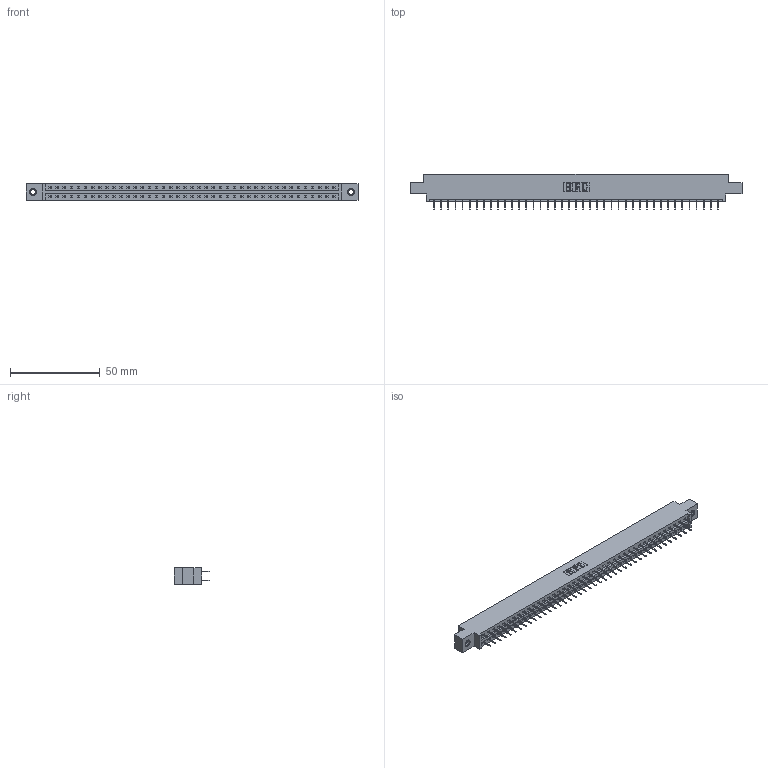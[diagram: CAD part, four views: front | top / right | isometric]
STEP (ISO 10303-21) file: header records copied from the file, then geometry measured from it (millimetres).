
FILE_DESCRIPTION (( 'STEP AP203' ), '1' );
FILE_NAME ('337-082-524-807.STEP', '2018-08-12T20:03:59', ( '' ), ( '' ), 'SwSTEP 2.0', 'SolidWorks 2016', '' );
FILE_SCHEMA (( 'CONFIG_CONTROL_DESIGN' ));
Length unit declared in the file: inch
Products named in the file (4): 345-250-001_345-250-005-103; 337-082-524-807; 337 Part_0.170 Offset - 0.156 Dia-TI; 345-292-001_345-293-124
Assembly tree (85 placements, depth 2):
  337-082-524-807
    337 Part_0.170 Offset - 0.156 Dia-TI
    345-292-001_345-293-124  x82
    345-250-001_345-250-005-103  x2
Bounding box: 185.47 x 19.69 x 9.4 mm (x, y, z)
Volume: 19278 mm3; surface area: 21543.5 mm2
Topology: 85 solids, 85 shells, 4934 faces, 13989 edges, 8990 vertices
Faces by surface type: plane 3714, cylinder 1204, cone 12, torus 4
Entity records: 33310 total; most frequent: CARTESIAN_POINT 5593, ORIENTED_EDGE 5522, DIRECTION 4791, EDGE_CURVE 2761, LINE 2617, VECTOR 2617, VERTEX_POINT 1832, AXIS2_PLACEMENT_3D 1087
